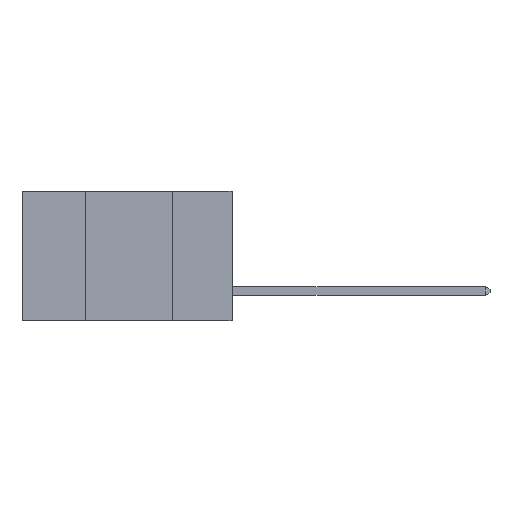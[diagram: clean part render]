
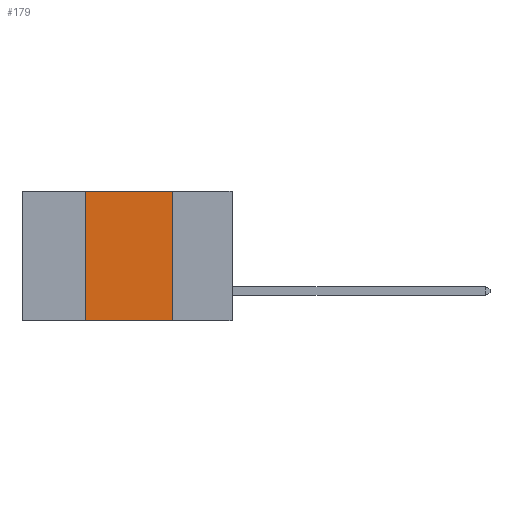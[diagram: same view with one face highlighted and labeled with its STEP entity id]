
A CAD part, left-side view. The second image highlights one B-rep face of the part: STEP entity #179.
In plain terms, the highlighted planar face has unit normal (-1, 0, 0).
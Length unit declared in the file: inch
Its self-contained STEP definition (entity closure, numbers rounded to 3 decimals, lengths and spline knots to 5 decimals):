
#179 = ADVANCED_FACE ( 'NONE', ( #5941 ), #6986, .F. ) ;
#1230 = CARTESIAN_POINT ( 'NONE',  ( 0., 0.17, -0.37 ) ) ;
#1723 = LINE ( 'NONE', #22516, #19533 ) ;
#1754 = LINE ( 'NONE', #5184, #16483 ) ;
#2817 = EDGE_CURVE ( 'NONE', #22119, #4878, #1723, .T. ) ;
#3319 = ORIENTED_EDGE ( 'NONE', *, *, #10609, .F. ) ;
#4199 = CARTESIAN_POINT ( 'NONE',  ( 0., 0.42, -0.37 ) ) ;
#4514 = ORIENTED_EDGE ( 'NONE', *, *, #8121, .T. ) ;
#4671 = EDGE_LOOP ( 'NONE', ( #21083, #16861, #3319, #4514 ) ) ;
#4878 = VERTEX_POINT ( 'NONE', #17853 ) ;
#5184 = CARTESIAN_POINT ( 'NONE',  ( 0., 0.17, 0. ) ) ;
#5941 = FACE_OUTER_BOUND ( 'NONE', #4671, .T. ) ;
#6236 = LINE ( 'NONE', #20235, #10567 ) ;
#6914 = LINE ( 'NONE', #21493, #16049 ) ;
#6986 = PLANE ( 'NONE',  #21755 ) ;
#8121 = EDGE_CURVE ( 'NONE', #17353, #14238, #6236, .T. ) ;
#10009 = DIRECTION ( 'NONE',  ( 1., 0., 0. ) ) ;
#10507 = CARTESIAN_POINT ( 'NONE',  ( 0., 0.6, 0. ) ) ;
#10567 = VECTOR ( 'NONE', #22028, 39.37008 ) ;
#10609 = EDGE_CURVE ( 'NONE', #17353, #22119, #6914, .T. ) ;
#11471 = CARTESIAN_POINT ( 'NONE',  ( 0., 0.42, 0. ) ) ;
#12707 = DIRECTION ( 'NONE',  ( 0., 0., -1. ) ) ;
#14238 = VERTEX_POINT ( 'NONE', #1230 ) ;
#14254 = EDGE_CURVE ( 'NONE', #4878, #14238, #1754, .T. ) ;
#16049 = VECTOR ( 'NONE', #23273, 39.37008 ) ;
#16483 = VECTOR ( 'NONE', #17967, 39.37008 ) ;
#16861 = ORIENTED_EDGE ( 'NONE', *, *, #2817, .F. ) ;
#17353 = VERTEX_POINT ( 'NONE', #4199 ) ;
#17853 = CARTESIAN_POINT ( 'NONE',  ( 0., 0.17, 0. ) ) ;
#17967 = DIRECTION ( 'NONE',  ( 0., 0., -1. ) ) ;
#19533 = VECTOR ( 'NONE', #22822, 39.37008 ) ;
#20235 = CARTESIAN_POINT ( 'NONE',  ( 0., 0.6, -0.37 ) ) ;
#21083 = ORIENTED_EDGE ( 'NONE', *, *, #14254, .F. ) ;
#21493 = CARTESIAN_POINT ( 'NONE',  ( 0., 0.42, 0. ) ) ;
#21755 = AXIS2_PLACEMENT_3D ( 'NONE', #10507, #10009, #12707 ) ;
#22028 = DIRECTION ( 'NONE',  ( 0., -1., 0. ) ) ;
#22119 = VERTEX_POINT ( 'NONE', #11471 ) ;
#22516 = CARTESIAN_POINT ( 'NONE',  ( 0., 0.6, 0. ) ) ;
#22822 = DIRECTION ( 'NONE',  ( 0., -1., 0. ) ) ;
#23273 = DIRECTION ( 'NONE',  ( 0., 0., 1. ) ) ;
